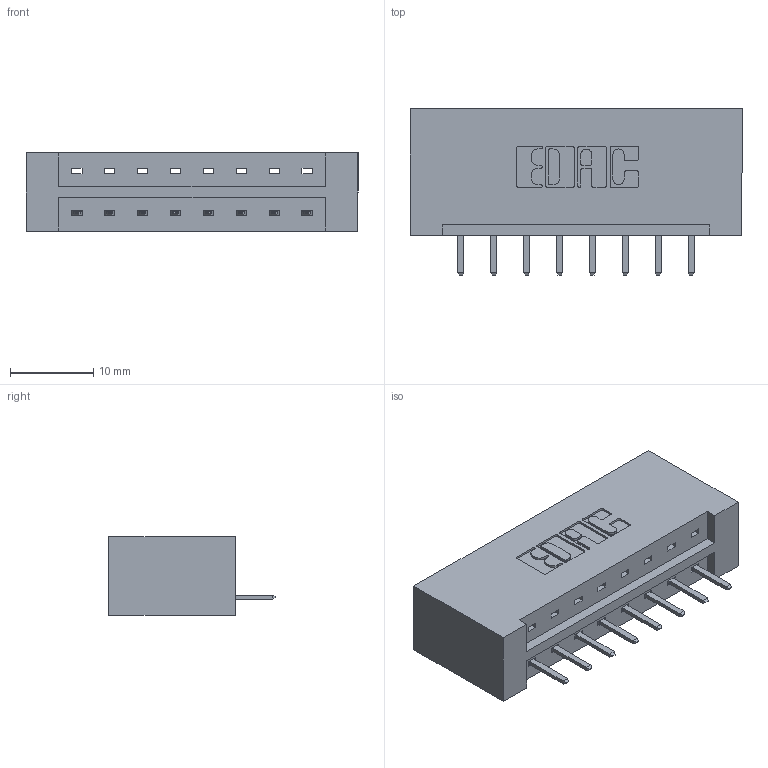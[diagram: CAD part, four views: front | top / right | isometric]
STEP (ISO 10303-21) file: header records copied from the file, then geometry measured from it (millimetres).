
FILE_DESCRIPTION (( 'STEP AP203' ), '1' );
FILE_NAME ('333-008-520-101.STEP', '2018-07-31T21:53:41', ( '' ), ( '' ), 'SwSTEP 2.0', 'SolidWorks 2016', '' );
FILE_SCHEMA (( 'CONFIG_CONTROL_DESIGN' ));
Length unit declared in the file: inch
Products named in the file (3): 333 Part_Lugless; 345-292-001_345-293-120; 333-008-520-101
Assembly tree (9 placements, depth 2):
  333-008-520-101
    333 Part_Lugless
    345-292-001_345-293-120  x8
Bounding box: 39.95 x 20.02 x 9.4 mm (x, y, z)
Volume: 4317.9 mm3; surface area: 4325.1 mm2
Topology: 9 solids, 9 shells, 602 faces, 1759 edges, 1150 vertices
Faces by surface type: plane 418, cylinder 184
Entity records: 9125 total; most frequent: CARTESIAN_POINT 1598, ORIENTED_EDGE 1530, DIRECTION 1397, EDGE_CURVE 765, LINE 641, VECTOR 641, VERTEX_POINT 506, AXIS2_PLACEMENT_3D 378
